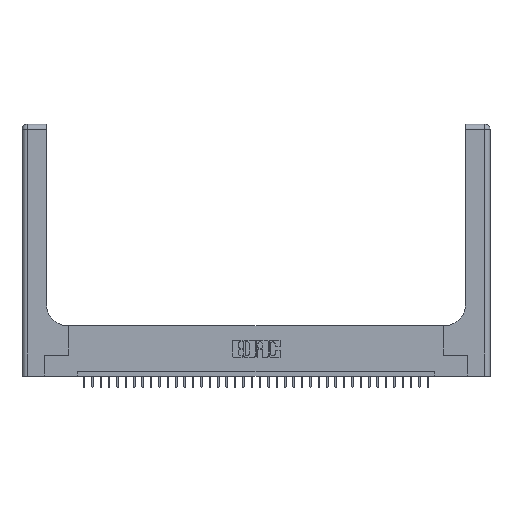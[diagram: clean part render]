
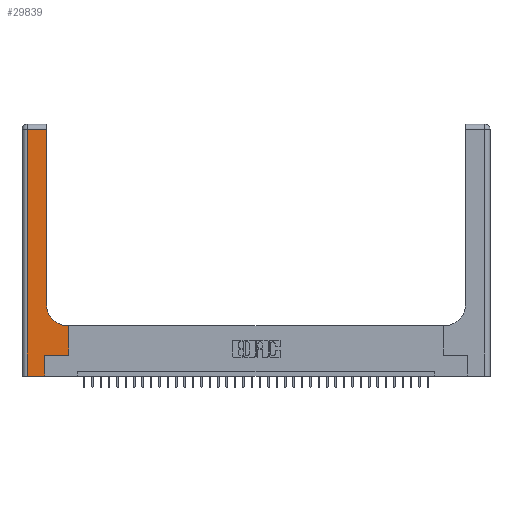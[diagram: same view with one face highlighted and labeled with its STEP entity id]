
A CAD part, top view. The second image highlights one B-rep face of the part: STEP entity #29839.
In plain terms, the highlighted planar face has unit normal (0, 0, 1).
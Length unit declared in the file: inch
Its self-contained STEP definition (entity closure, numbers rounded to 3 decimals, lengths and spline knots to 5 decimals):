
#347 = FACE_OUTER_BOUND ( 'NONE', #18824, .T. ) ;
#1157 = CARTESIAN_POINT ( 'NONE',  ( 0., 2.94, 0.37 ) ) ;
#1205 = VECTOR ( 'NONE', #35075, 39.37008 ) ;
#1890 = VECTOR ( 'NONE', #35311, 39.37008 ) ;
#3242 = CARTESIAN_POINT ( 'NONE',  ( 0.269, 0.25, 0.37 ) ) ;
#3371 = DIRECTION ( 'NONE',  ( 0., -1., 0. ) ) ;
#3376 = DIRECTION ( 'NONE',  ( 1., 0., 0. ) ) ;
#3953 = LINE ( 'NONE', #1157, #1890 ) ;
#4122 = CARTESIAN_POINT ( 'NONE',  ( 0.5415, 0.6, 0.37 ) ) ;
#4202 = AXIS2_PLACEMENT_3D ( 'NONE', #17124, #26054, #22908 ) ;
#4268 = VERTEX_POINT ( 'NONE', #25146 ) ;
#4584 = CARTESIAN_POINT ( 'NONE',  ( 0.5415, 0.85, 0.37 ) ) ;
#4742 = VERTEX_POINT ( 'NONE', #31618 ) ;
#5201 = EDGE_CURVE ( 'NONE', #34342, #7930, #17732, .T. ) ;
#5889 = CARTESIAN_POINT ( 'NONE',  ( 0.5585, 0.25, 0.37 ) ) ;
#6172 = CARTESIAN_POINT ( 'NONE',  ( 0.06, 0., 0.37 ) ) ;
#7764 = EDGE_CURVE ( 'NONE', #30613, #9642, #34734, .T. ) ;
#7930 = VERTEX_POINT ( 'NONE', #31598 ) ;
#7964 = VECTOR ( 'NONE', #35321, 39.37008 ) ;
#8111 = ORIENTED_EDGE ( 'NONE', *, *, #10422, .T. ) ;
#8322 = LINE ( 'NONE', #31111, #9400 ) ;
#8841 = DIRECTION ( 'NONE',  ( 0., 1., 0. ) ) ;
#8894 = DIRECTION ( 'NONE',  ( 1., 0., 0. ) ) ;
#9376 = EDGE_CURVE ( 'NONE', #4268, #34342, #30254, .T. ) ;
#9400 = VECTOR ( 'NONE', #8894, 39.37008 ) ;
#9642 = VERTEX_POINT ( 'NONE', #6172 ) ;
#10422 = EDGE_CURVE ( 'NONE', #7930, #11517, #14674, .T. ) ;
#10948 = CARTESIAN_POINT ( 'NONE',  ( 0.5585, 0.6, 0.37 ) ) ;
#11517 = VERTEX_POINT ( 'NONE', #10948 ) ;
#11781 = CARTESIAN_POINT ( 'NONE',  ( 0.06, 3., 0.37 ) ) ;
#12216 = ORIENTED_EDGE ( 'NONE', *, *, #29547, .T. ) ;
#12305 = ORIENTED_EDGE ( 'NONE', *, *, #7764, .T. ) ;
#12583 = ORIENTED_EDGE ( 'NONE', *, *, #9376, .T. ) ;
#13027 = ORIENTED_EDGE ( 'NONE', *, *, #5201, .T. ) ;
#14674 = LINE ( 'NONE', #5889, #7964 ) ;
#14986 = LINE ( 'NONE', #31803, #23986 ) ;
#15289 = LINE ( 'NONE', #15841, #1205 ) ;
#15841 = CARTESIAN_POINT ( 'NONE',  ( 0.2915, 0.6, 0.37 ) ) ;
#15971 = DIRECTION ( 'NONE',  ( 1., 0., 0. ) ) ;
#16875 = VECTOR ( 'NONE', #3371, 39.37008 ) ;
#17124 = CARTESIAN_POINT ( 'NONE',  ( 0., 3., 0.37 ) ) ;
#17382 = VERTEX_POINT ( 'NONE', #4122 ) ;
#17732 = LINE ( 'NONE', #28937, #22687 ) ;
#18824 = EDGE_LOOP ( 'NONE', ( #29450, #21911, #12305, #21322, #12583, #13027, #8111, #12216, #34390 ) ) ;
#19179 = AXIS2_PLACEMENT_3D ( 'NONE', #4584, #30537, #15971 ) ;
#19710 = EDGE_CURVE ( 'NONE', #36305, #30613, #3953, .T. ) ;
#20097 = EDGE_CURVE ( 'NONE', #17382, #4742, #25730, .T. ) ;
#20475 = PLANE ( 'NONE',  #4202 ) ;
#21322 = ORIENTED_EDGE ( 'NONE', *, *, #26588, .T. ) ;
#21911 = ORIENTED_EDGE ( 'NONE', *, *, #19710, .T. ) ;
#22687 = VECTOR ( 'NONE', #3376, 39.37008 ) ;
#22908 = DIRECTION ( 'NONE',  ( -1., 0., 0. ) ) ;
#23986 = VECTOR ( 'NONE', #8841, 39.37008 ) ;
#24450 = CARTESIAN_POINT ( 'NONE',  ( 0.269, 0., 0.37 ) ) ;
#25146 = CARTESIAN_POINT ( 'NONE',  ( 0.269, 0., 0.37 ) ) ;
#25730 = CIRCLE ( 'NONE', #19179, 0.25 ) ;
#26054 = DIRECTION ( 'NONE',  ( 0., 0., -1. ) ) ;
#26588 = EDGE_CURVE ( 'NONE', #9642, #4268, #8322, .T. ) ;
#28546 = CARTESIAN_POINT ( 'NONE',  ( 0.06, 2.94, 0.37 ) ) ;
#28937 = CARTESIAN_POINT ( 'NONE',  ( 0.269, 0.25, 0.37 ) ) ;
#29450 = ORIENTED_EDGE ( 'NONE', *, *, #34408, .T. ) ;
#29547 = EDGE_CURVE ( 'NONE', #11517, #17382, #15289, .T. ) ;
#29696 = DIRECTION ( 'NONE',  ( 0., 1., 0. ) ) ;
#29839 = ADVANCED_FACE ( 'NONE', ( #347 ), #20475, .F. ) ;
#30254 = LINE ( 'NONE', #24450, #34259 ) ;
#30537 = DIRECTION ( 'NONE',  ( 0., 0., -1. ) ) ;
#30613 = VERTEX_POINT ( 'NONE', #28546 ) ;
#31111 = CARTESIAN_POINT ( 'NONE',  ( 0., 0., 0.37 ) ) ;
#31407 = CARTESIAN_POINT ( 'NONE',  ( 0.2915, 2.94, 0.37 ) ) ;
#31598 = CARTESIAN_POINT ( 'NONE',  ( 0.5585, 0.25, 0.37 ) ) ;
#31618 = CARTESIAN_POINT ( 'NONE',  ( 0.2915, 0.85, 0.37 ) ) ;
#31803 = CARTESIAN_POINT ( 'NONE',  ( 0.2915, 3., 0.37 ) ) ;
#34259 = VECTOR ( 'NONE', #29696, 39.37008 ) ;
#34342 = VERTEX_POINT ( 'NONE', #3242 ) ;
#34390 = ORIENTED_EDGE ( 'NONE', *, *, #20097, .T. ) ;
#34408 = EDGE_CURVE ( 'NONE', #4742, #36305, #14986, .T. ) ;
#34734 = LINE ( 'NONE', #11781, #16875 ) ;
#35075 = DIRECTION ( 'NONE',  ( -1., 0., 0. ) ) ;
#35311 = DIRECTION ( 'NONE',  ( -1., 0., 0. ) ) ;
#35321 = DIRECTION ( 'NONE',  ( 0., 1., 0. ) ) ;
#36305 = VERTEX_POINT ( 'NONE', #31407 ) ;
